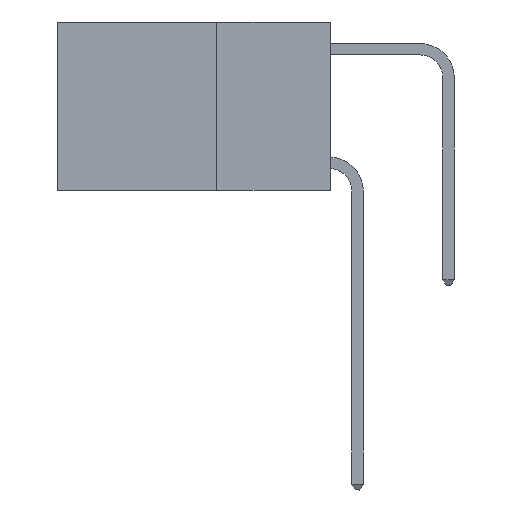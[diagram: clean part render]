
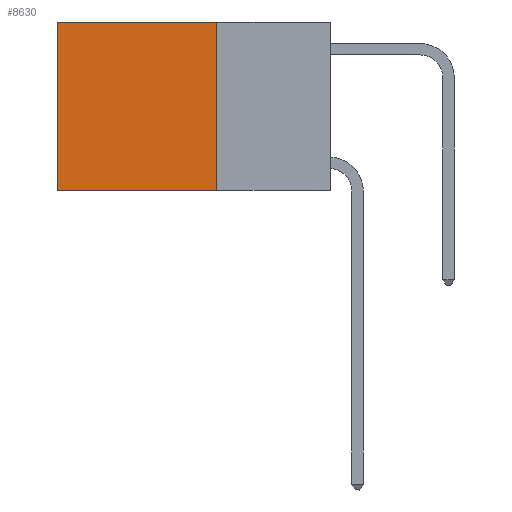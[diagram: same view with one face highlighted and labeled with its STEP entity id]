
A CAD part, left-side view. The second image highlights one B-rep face of the part: STEP entity #8630.
In plain terms, the highlighted planar face has unit normal (-1, 0, 0).
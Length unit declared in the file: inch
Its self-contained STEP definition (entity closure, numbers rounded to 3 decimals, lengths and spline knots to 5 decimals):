
#254 = LINE ( 'NONE', #8131, #5922 ) ;
#306 = LINE ( 'NONE', #4689, #5651 ) ;
#982 = VERTEX_POINT ( 'NONE', #11677 ) ;
#1081 = PLANE ( 'NONE',  #1180 ) ;
#1180 = AXIS2_PLACEMENT_3D ( 'NONE', #5270, #8282, #2166 ) ;
#2009 = DIRECTION ( 'NONE',  ( 0., 0., -1. ) ) ;
#2166 = DIRECTION ( 'NONE',  ( 0., 0., -1. ) ) ;
#2309 = DIRECTION ( 'NONE',  ( 0., 1., 0. ) ) ;
#2606 = FACE_OUTER_BOUND ( 'NONE', #8809, .T. ) ;
#2725 = EDGE_CURVE ( 'NONE', #12132, #9040, #254, .T. ) ;
#3038 = DIRECTION ( 'NONE',  ( 0., 1., 0. ) ) ;
#3751 = VERTEX_POINT ( 'NONE', #6335 ) ;
#4415 = CARTESIAN_POINT ( 'NONE',  ( 0.2625, 0.25, -0.37 ) ) ;
#4689 = CARTESIAN_POINT ( 'NONE',  ( 0.2625, 0.6, 0. ) ) ;
#5270 = CARTESIAN_POINT ( 'NONE',  ( 0.2625, 0.25, 0. ) ) ;
#5651 = VECTOR ( 'NONE', #5688, 39.37008 ) ;
#5688 = DIRECTION ( 'NONE',  ( 0., 0., -1. ) ) ;
#5922 = VECTOR ( 'NONE', #2009, 39.37008 ) ;
#6335 = CARTESIAN_POINT ( 'NONE',  ( 0.2625, 0.6, -0.37 ) ) ;
#7027 = VECTOR ( 'NONE', #2309, 39.37008 ) ;
#8131 = CARTESIAN_POINT ( 'NONE',  ( 0.2625, 0.25, 0. ) ) ;
#8282 = DIRECTION ( 'NONE',  ( 1., 0., 0. ) ) ;
#8303 = LINE ( 'NONE', #12890, #10624 ) ;
#8630 = ADVANCED_FACE ( 'NONE', ( #2606 ), #1081, .F. ) ;
#8809 = EDGE_LOOP ( 'NONE', ( #9393, #9449, #9633, #9662 ) ) ;
#9040 = VERTEX_POINT ( 'NONE', #11804 ) ;
#9393 = ORIENTED_EDGE ( 'NONE', *, *, #11984, .T. ) ;
#9449 = ORIENTED_EDGE ( 'NONE', *, *, #12633, .F. ) ;
#9633 = ORIENTED_EDGE ( 'NONE', *, *, #2725, .F. ) ;
#9662 = ORIENTED_EDGE ( 'NONE', *, *, #11452, .T. ) ;
#10624 = VECTOR ( 'NONE', #3038, 39.37008 ) ;
#10814 = CARTESIAN_POINT ( 'NONE',  ( 0.2625, 0.25, 0. ) ) ;
#11452 = EDGE_CURVE ( 'NONE', #12132, #982, #8303, .T. ) ;
#11677 = CARTESIAN_POINT ( 'NONE',  ( 0.2625, 0.6, 0. ) ) ;
#11804 = CARTESIAN_POINT ( 'NONE',  ( 0.2625, 0.25, -0.37 ) ) ;
#11984 = EDGE_CURVE ( 'NONE', #982, #3751, #306, .T. ) ;
#12132 = VERTEX_POINT ( 'NONE', #10814 ) ;
#12534 = LINE ( 'NONE', #4415, #7027 ) ;
#12633 = EDGE_CURVE ( 'NONE', #9040, #3751, #12534, .T. ) ;
#12890 = CARTESIAN_POINT ( 'NONE',  ( 0.2625, 0.25, 0. ) ) ;
